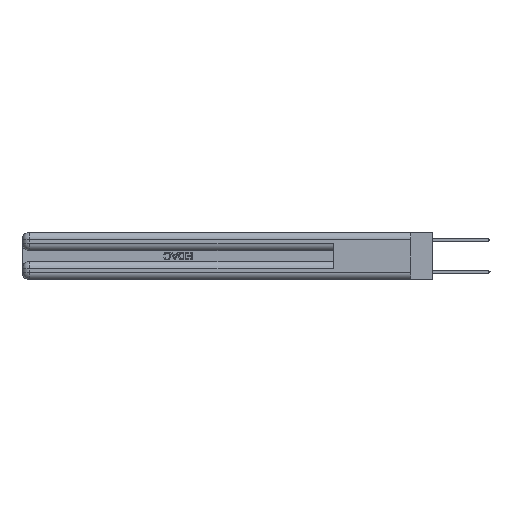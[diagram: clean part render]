
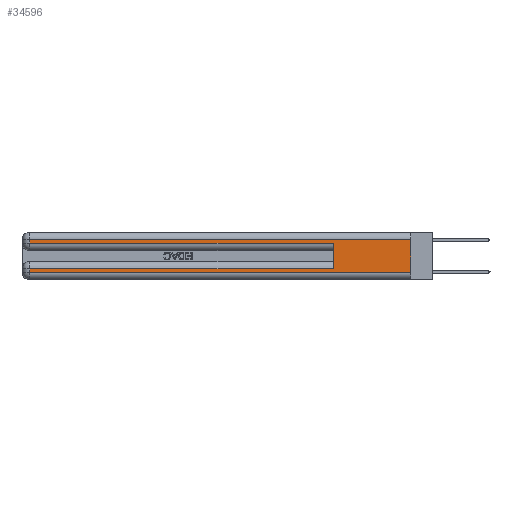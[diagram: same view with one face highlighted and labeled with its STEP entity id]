
A CAD part, left-side view. The second image highlights one B-rep face of the part: STEP entity #34596.
In plain terms, the highlighted planar face has unit normal (-1, 0, 0).
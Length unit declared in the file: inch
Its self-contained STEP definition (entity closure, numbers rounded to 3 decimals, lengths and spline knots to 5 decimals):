
#343 = DIRECTION ( 'NONE',  ( 0., 0., 1. ) ) ;
#996 = LINE ( 'NONE', #1732, #1102 ) ;
#1102 = VECTOR ( 'NONE', #24616, 39.37008 ) ;
#1565 = VERTEX_POINT ( 'NONE', #28507 ) ;
#1732 = CARTESIAN_POINT ( 'NONE',  ( 0., 0., 0.06 ) ) ;
#2373 = CARTESIAN_POINT ( 'NONE',  ( 0., 0., 0.37 ) ) ;
#2513 = FACE_OUTER_BOUND ( 'NONE', #7358, .T. ) ;
#2782 = CARTESIAN_POINT ( 'NONE',  ( 0., 2.94, 0.31 ) ) ;
#4072 = LINE ( 'NONE', #15598, #30544 ) ;
#4427 = EDGE_CURVE ( 'NONE', #27282, #8668, #13536, .T. ) ;
#4447 = VECTOR ( 'NONE', #34355, 39.37008 ) ;
#4728 = CARTESIAN_POINT ( 'NONE',  ( 0., 0., 0.31 ) ) ;
#4749 = ORIENTED_EDGE ( 'NONE', *, *, #9274, .T. ) ;
#5720 = LINE ( 'NONE', #36935, #36075 ) ;
#6242 = LINE ( 'NONE', #14382, #33301 ) ;
#6542 = DIRECTION ( 'NONE',  ( 0., 1., 0. ) ) ;
#6544 = ORIENTED_EDGE ( 'NONE', *, *, #17209, .F. ) ;
#7317 = VECTOR ( 'NONE', #27919, 39.37008 ) ;
#7358 = EDGE_LOOP ( 'NONE', ( #26794, #35955, #9684, #9662, #6544, #30062, #4749, #30418 ) ) ;
#8668 = VERTEX_POINT ( 'NONE', #8940 ) ;
#8940 = CARTESIAN_POINT ( 'NONE',  ( 0., 0., 0.06 ) ) ;
#9274 = EDGE_CURVE ( 'NONE', #1565, #10292, #6242, .T. ) ;
#9662 = ORIENTED_EDGE ( 'NONE', *, *, #16081, .T. ) ;
#9684 = ORIENTED_EDGE ( 'NONE', *, *, #27996, .T. ) ;
#10292 = VERTEX_POINT ( 'NONE', #22610 ) ;
#11303 = CARTESIAN_POINT ( 'NONE',  ( 0., 2.94, 0.37 ) ) ;
#11409 = CARTESIAN_POINT ( 'NONE',  ( 0., 0., 0.37 ) ) ;
#11596 = DIRECTION ( 'NONE',  ( 0., 0., -1. ) ) ;
#11700 = EDGE_CURVE ( 'NONE', #27282, #29324, #4072, .T. ) ;
#13536 = LINE ( 'NONE', #2373, #7317 ) ;
#14382 = CARTESIAN_POINT ( 'NONE',  ( 0., 2.94, 0.37 ) ) ;
#15598 = CARTESIAN_POINT ( 'NONE',  ( 0., 0., 0.31 ) ) ;
#15897 = EDGE_CURVE ( 'NONE', #26620, #1565, #32101, .T. ) ;
#16081 = EDGE_CURVE ( 'NONE', #34492, #24855, #5720, .T. ) ;
#16457 = EDGE_CURVE ( 'NONE', #10292, #8668, #996, .T. ) ;
#17209 = EDGE_CURVE ( 'NONE', #26620, #24855, #20381, .T. ) ;
#17468 = CARTESIAN_POINT ( 'NONE',  ( 0., 0.6, 0.085 ) ) ;
#18979 = CARTESIAN_POINT ( 'NONE',  ( 0., 2.94, 0.285 ) ) ;
#19009 = CARTESIAN_POINT ( 'NONE',  ( 0., 0.6, 0.285 ) ) ;
#20381 = LINE ( 'NONE', #26245, #22850 ) ;
#22554 = DIRECTION ( 'NONE',  ( 0., -1., 0. ) ) ;
#22610 = CARTESIAN_POINT ( 'NONE',  ( 0., 2.94, 0.06 ) ) ;
#22850 = VECTOR ( 'NONE', #343, 39.37008 ) ;
#24616 = DIRECTION ( 'NONE',  ( 0., -1., 0. ) ) ;
#24855 = VERTEX_POINT ( 'NONE', #19009 ) ;
#25595 = PLANE ( 'NONE',  #27639 ) ;
#26245 = CARTESIAN_POINT ( 'NONE',  ( 0., 0.6, 0.145 ) ) ;
#26620 = VERTEX_POINT ( 'NONE', #17468 ) ;
#26794 = ORIENTED_EDGE ( 'NONE', *, *, #4427, .F. ) ;
#27045 = VECTOR ( 'NONE', #31542, 39.37008 ) ;
#27282 = VERTEX_POINT ( 'NONE', #4728 ) ;
#27639 = AXIS2_PLACEMENT_3D ( 'NONE', #11409, #37115, #11596 ) ;
#27919 = DIRECTION ( 'NONE',  ( 0., 0., -1. ) ) ;
#27996 = EDGE_CURVE ( 'NONE', #29324, #34492, #37193, .T. ) ;
#28507 = CARTESIAN_POINT ( 'NONE',  ( 0., 2.94, 0.085 ) ) ;
#28522 = CARTESIAN_POINT ( 'NONE',  ( 0., 0., 0.085 ) ) ;
#29324 = VERTEX_POINT ( 'NONE', #2782 ) ;
#30062 = ORIENTED_EDGE ( 'NONE', *, *, #15897, .T. ) ;
#30418 = ORIENTED_EDGE ( 'NONE', *, *, #16457, .T. ) ;
#30544 = VECTOR ( 'NONE', #6542, 39.37008 ) ;
#31542 = DIRECTION ( 'NONE',  ( 0., 1., 0. ) ) ;
#32101 = LINE ( 'NONE', #28522, #27045 ) ;
#32150 = DIRECTION ( 'NONE',  ( 0., 0., -1. ) ) ;
#33301 = VECTOR ( 'NONE', #32150, 39.37008 ) ;
#34355 = DIRECTION ( 'NONE',  ( 0., 0., -1. ) ) ;
#34492 = VERTEX_POINT ( 'NONE', #18979 ) ;
#34596 = ADVANCED_FACE ( 'NONE', ( #2513 ), #25595, .F. ) ;
#35955 = ORIENTED_EDGE ( 'NONE', *, *, #11700, .T. ) ;
#36075 = VECTOR ( 'NONE', #22554, 39.37008 ) ;
#36935 = CARTESIAN_POINT ( 'NONE',  ( 0., 0., 0.285 ) ) ;
#37115 = DIRECTION ( 'NONE',  ( 1., 0., 0. ) ) ;
#37193 = LINE ( 'NONE', #11303, #4447 ) ;
